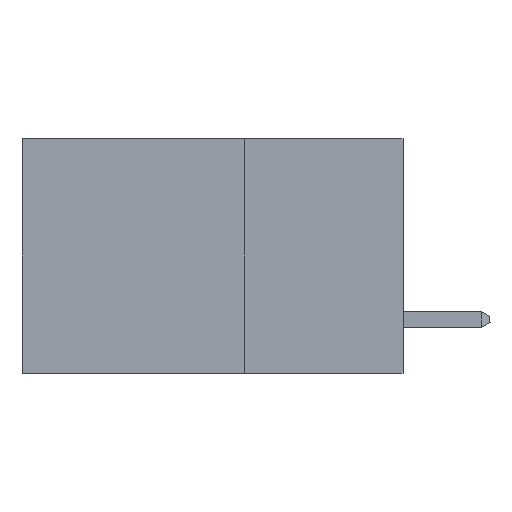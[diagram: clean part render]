
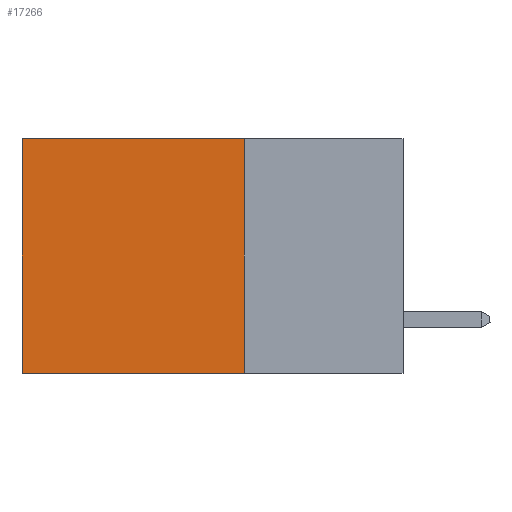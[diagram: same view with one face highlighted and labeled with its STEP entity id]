
A CAD part, left-side view. The second image highlights one B-rep face of the part: STEP entity #17266.
In plain terms, the highlighted planar face has unit normal (-1, 0, 0).
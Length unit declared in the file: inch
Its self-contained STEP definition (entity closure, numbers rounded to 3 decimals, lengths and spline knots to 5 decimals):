
#502 = EDGE_CURVE ( 'NONE', #3765, #2737, #14455, .T. ) ;
#2009 = EDGE_CURVE ( 'NONE', #45975, #3765, #19974, .T. ) ;
#2581 = CARTESIAN_POINT ( 'NONE',  ( 0.2875, 0.6, 0. ) ) ;
#2737 = VERTEX_POINT ( 'NONE', #10369 ) ;
#2898 = ORIENTED_EDGE ( 'NONE', *, *, #2009, .F. ) ;
#3765 = VERTEX_POINT ( 'NONE', #6273 ) ;
#6273 = CARTESIAN_POINT ( 'NONE',  ( 0.2875, 0.25, -0.37 ) ) ;
#8094 = DIRECTION ( 'NONE',  ( 0., 0., -1. ) ) ;
#9815 = VECTOR ( 'NONE', #35450, 39.37008 ) ;
#10172 = VECTOR ( 'NONE', #44476, 39.37008 ) ;
#10369 = CARTESIAN_POINT ( 'NONE',  ( 0.2875, 0.6, -0.37 ) ) ;
#12130 = PLANE ( 'NONE',  #44444 ) ;
#12461 = DIRECTION ( 'NONE',  ( 1., 0., 0. ) ) ;
#12521 = ORIENTED_EDGE ( 'NONE', *, *, #502, .F. ) ;
#14455 = LINE ( 'NONE', #33679, #32917 ) ;
#17073 = LINE ( 'NONE', #39419, #21191 ) ;
#17266 = ADVANCED_FACE ( 'NONE', ( #23948 ), #12130, .F. ) ;
#19776 = CARTESIAN_POINT ( 'NONE',  ( 0.2875, 0.25, 0. ) ) ;
#19974 = LINE ( 'NONE', #19776, #9815 ) ;
#21191 = VECTOR ( 'NONE', #39259, 39.37008 ) ;
#23948 = FACE_OUTER_BOUND ( 'NONE', #47551, .T. ) ;
#25982 = CARTESIAN_POINT ( 'NONE',  ( 0.2875, 0.25, 0. ) ) ;
#27423 = VERTEX_POINT ( 'NONE', #40724 ) ;
#29352 = DIRECTION ( 'NONE',  ( 0., 1., 0. ) ) ;
#29743 = EDGE_CURVE ( 'NONE', #27423, #2737, #31681, .T. ) ;
#31681 = LINE ( 'NONE', #2581, #10172 ) ;
#32917 = VECTOR ( 'NONE', #29352, 39.37008 ) ;
#33679 = CARTESIAN_POINT ( 'NONE',  ( 0.2875, 0.25, -0.37 ) ) ;
#35317 = CARTESIAN_POINT ( 'NONE',  ( 0.2875, 0.25, 0. ) ) ;
#35450 = DIRECTION ( 'NONE',  ( 0., 0., -1. ) ) ;
#37382 = EDGE_CURVE ( 'NONE', #45975, #27423, #17073, .T. ) ;
#39259 = DIRECTION ( 'NONE',  ( 0., 1., 0. ) ) ;
#39419 = CARTESIAN_POINT ( 'NONE',  ( 0.2875, 0.25, 0. ) ) ;
#40724 = CARTESIAN_POINT ( 'NONE',  ( 0.2875, 0.6, 0. ) ) ;
#44072 = ORIENTED_EDGE ( 'NONE', *, *, #29743, .T. ) ;
#44444 = AXIS2_PLACEMENT_3D ( 'NONE', #35317, #12461, #8094 ) ;
#44476 = DIRECTION ( 'NONE',  ( 0., 0., -1. ) ) ;
#45975 = VERTEX_POINT ( 'NONE', #25982 ) ;
#47551 = EDGE_LOOP ( 'NONE', ( #44072, #12521, #2898, #48814 ) ) ;
#48814 = ORIENTED_EDGE ( 'NONE', *, *, #37382, .T. ) ;
